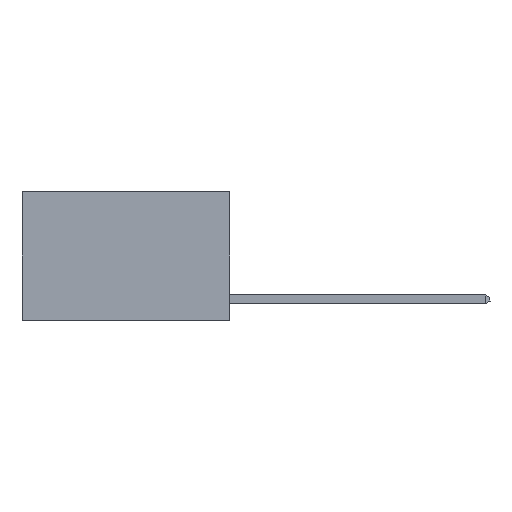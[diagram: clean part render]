
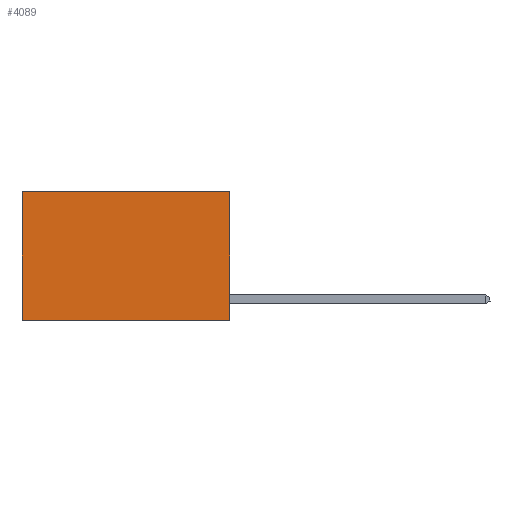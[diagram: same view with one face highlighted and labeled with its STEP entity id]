
A CAD part, left-side view. The second image highlights one B-rep face of the part: STEP entity #4089.
In plain terms, the highlighted planar face has unit normal (-1, 0, 0).
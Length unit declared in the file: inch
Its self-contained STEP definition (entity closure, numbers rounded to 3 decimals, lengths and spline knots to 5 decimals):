
#397 = DIRECTION ( 'NONE',  ( 0., 0., -1. ) ) ;
#657 = DIRECTION ( 'NONE',  ( 0., 1., 0. ) ) ;
#736 = CARTESIAN_POINT ( 'NONE',  ( 0.2625, 0., -0.37 ) ) ;
#1352 = CARTESIAN_POINT ( 'NONE',  ( 0.2625, 0.6, 0. ) ) ;
#1369 = CARTESIAN_POINT ( 'NONE',  ( 0.2625, 0., 0. ) ) ;
#1828 = ORIENTED_EDGE ( 'NONE', *, *, #11395, .T. ) ;
#1958 = VECTOR ( 'NONE', #5681, 39.37008 ) ;
#2030 = EDGE_CURVE ( 'NONE', #5258, #6801, #8877, .T. ) ;
#2976 = FACE_OUTER_BOUND ( 'NONE', #3037, .T. ) ;
#3037 = EDGE_LOOP ( 'NONE', ( #12417, #7669, #8633, #1828 ) ) ;
#3224 = DIRECTION ( 'NONE',  ( 0., 0., -1. ) ) ;
#3648 = VERTEX_POINT ( 'NONE', #7811 ) ;
#4089 = ADVANCED_FACE ( 'NONE', ( #2976 ), #6328, .F. ) ;
#5258 = VERTEX_POINT ( 'NONE', #7802 ) ;
#5525 = LINE ( 'NONE', #9410, #6806 ) ;
#5681 = DIRECTION ( 'NONE',  ( 0., 1., 0. ) ) ;
#5724 = AXIS2_PLACEMENT_3D ( 'NONE', #7462, #12247, #8409 ) ;
#5777 = VERTEX_POINT ( 'NONE', #10690 ) ;
#6328 = PLANE ( 'NONE',  #5724 ) ;
#6635 = LINE ( 'NONE', #736, #1958 ) ;
#6801 = VERTEX_POINT ( 'NONE', #12698 ) ;
#6806 = VECTOR ( 'NONE', #657, 39.37008 ) ;
#7462 = CARTESIAN_POINT ( 'NONE',  ( 0.2625, 0., 0. ) ) ;
#7669 = ORIENTED_EDGE ( 'NONE', *, *, #8528, .F. ) ;
#7802 = CARTESIAN_POINT ( 'NONE',  ( 0.2625, 0.6, 0. ) ) ;
#7811 = CARTESIAN_POINT ( 'NONE',  ( 0.2625, 0., 0. ) ) ;
#8409 = DIRECTION ( 'NONE',  ( 0., 0., -1. ) ) ;
#8528 = EDGE_CURVE ( 'NONE', #5777, #6801, #6635, .T. ) ;
#8633 = ORIENTED_EDGE ( 'NONE', *, *, #8711, .F. ) ;
#8711 = EDGE_CURVE ( 'NONE', #3648, #5777, #9811, .T. ) ;
#8877 = LINE ( 'NONE', #1352, #10974 ) ;
#9100 = VECTOR ( 'NONE', #397, 39.37008 ) ;
#9410 = CARTESIAN_POINT ( 'NONE',  ( 0.2625, 0., 0. ) ) ;
#9811 = LINE ( 'NONE', #1369, #9100 ) ;
#10690 = CARTESIAN_POINT ( 'NONE',  ( 0.2625, 0., -0.37 ) ) ;
#10974 = VECTOR ( 'NONE', #3224, 39.37008 ) ;
#11395 = EDGE_CURVE ( 'NONE', #3648, #5258, #5525, .T. ) ;
#12247 = DIRECTION ( 'NONE',  ( 1., 0., 0. ) ) ;
#12417 = ORIENTED_EDGE ( 'NONE', *, *, #2030, .T. ) ;
#12698 = CARTESIAN_POINT ( 'NONE',  ( 0.2625, 0.6, -0.37 ) ) ;
